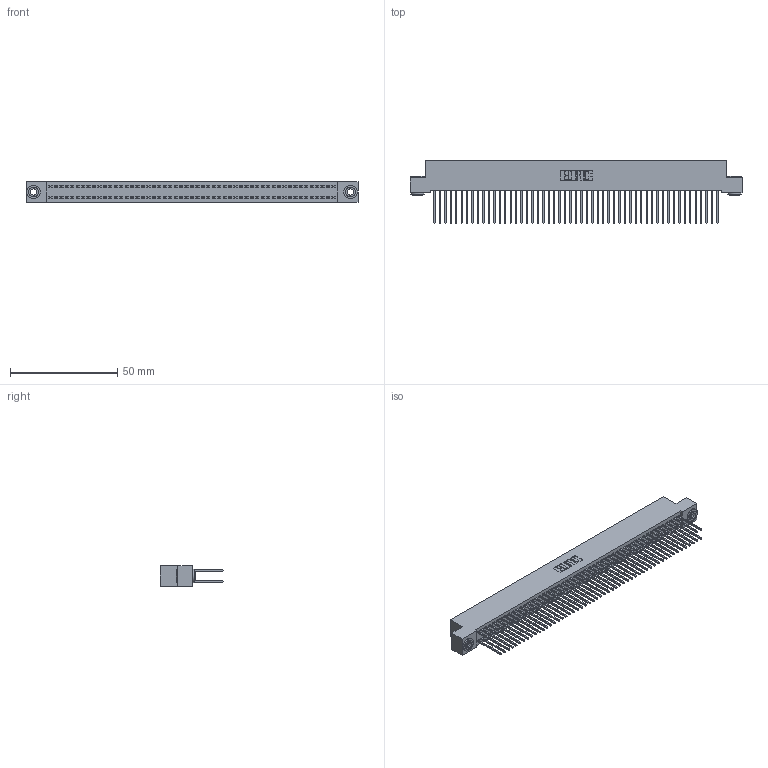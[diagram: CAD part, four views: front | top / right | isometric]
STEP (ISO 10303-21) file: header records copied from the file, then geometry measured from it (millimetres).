
FILE_DESCRIPTION (( 'STEP AP203' ), '1' );
FILE_NAME ('392-106-540-203.STEP', '2018-08-18T20:14:43', ( '' ), ( '' ), 'SwSTEP 2.0', 'SolidWorks 2016', '' );
FILE_SCHEMA (( 'CONFIG_CONTROL_DESIGN' ));
Length unit declared in the file: inch
Products named in the file (4): 342 Part_.156 TH; 345-292-001_345-293-140; 342-250-002_345-250-002-102; 392-106-540-203
Assembly tree (109 placements, depth 2):
  392-106-540-203
    342 Part_.156 TH
    345-292-001_345-293-140  x106
    342-250-002_345-250-002-102  x2
Bounding box: 154.94 x 29.47 x 9.4 mm (x, y, z)
Volume: 14398.1 mm3; surface area: 25708 mm2
Topology: 109 solids, 109 shells, 5660 faces, 16805 edges, 11058 vertices
Faces by surface type: plane 3892, cylinder 1760, cone 8
Entity records: 33210 total; most frequent: CARTESIAN_POINT 5465, ORIENTED_EDGE 5394, DIRECTION 4683, EDGE_CURVE 2697, VECTOR 2545, LINE 2545, VERTEX_POINT 1794, AXIS2_PLACEMENT_3D 1069
